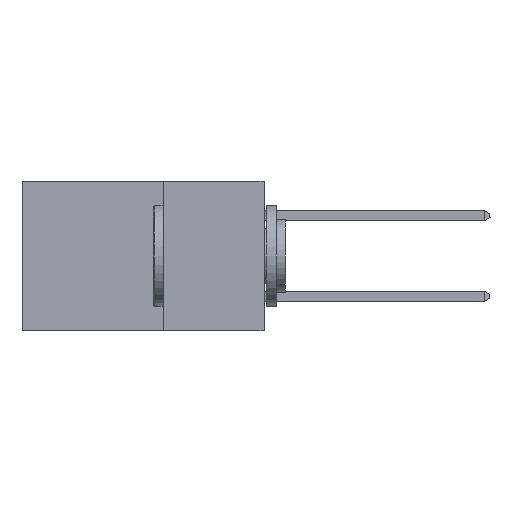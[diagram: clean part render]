
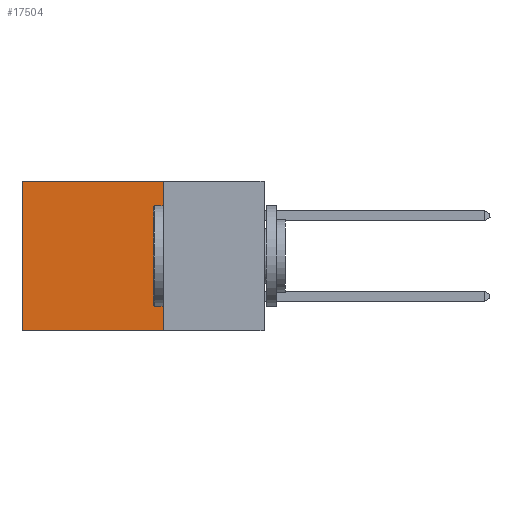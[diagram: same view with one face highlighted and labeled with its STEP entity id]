
A CAD part, left-side view. The second image highlights one B-rep face of the part: STEP entity #17504.
In plain terms, the highlighted planar face has unit normal (-1, 0, 0).
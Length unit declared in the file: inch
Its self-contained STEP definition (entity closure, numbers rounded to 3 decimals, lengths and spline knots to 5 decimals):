
#246 = CARTESIAN_POINT ( 'NONE',  ( 0.298, 0.6, 0. ) ) ;
#4098 = DIRECTION ( 'NONE',  ( 0., 1., 0. ) ) ;
#4342 = LINE ( 'NONE', #7445, #29197 ) ;
#4392 = CARTESIAN_POINT ( 'NONE',  ( 0.298, 0.25, -0.37 ) ) ;
#4753 = ORIENTED_EDGE ( 'NONE', *, *, #19702, .T. ) ;
#7445 = CARTESIAN_POINT ( 'NONE',  ( 0.298, 0.25, 0. ) ) ;
#9048 = VECTOR ( 'NONE', #27090, 39.37008 ) ;
#9497 = LINE ( 'NONE', #11102, #12648 ) ;
#10678 = ORIENTED_EDGE ( 'NONE', *, *, #26498, .T. ) ;
#10908 = PLANE ( 'NONE',  #15287 ) ;
#11012 = CARTESIAN_POINT ( 'NONE',  ( 0.298, 0.25, 0. ) ) ;
#11102 = CARTESIAN_POINT ( 'NONE',  ( 0.298, 0.25, 0. ) ) ;
#12343 = EDGE_CURVE ( 'NONE', #18523, #13558, #13963, .T. ) ;
#12648 = VECTOR ( 'NONE', #4098, 39.37008 ) ;
#13558 = VERTEX_POINT ( 'NONE', #21492 ) ;
#13963 = LINE ( 'NONE', #4392, #9048 ) ;
#14681 = CARTESIAN_POINT ( 'NONE',  ( 0.298, 0.6, 0. ) ) ;
#15287 = AXIS2_PLACEMENT_3D ( 'NONE', #11012, #15636, #27094 ) ;
#15636 = DIRECTION ( 'NONE',  ( 1., 0., 0. ) ) ;
#16677 = VERTEX_POINT ( 'NONE', #14681 ) ;
#16897 = VECTOR ( 'NONE', #22634, 39.37008 ) ;
#16905 = ORIENTED_EDGE ( 'NONE', *, *, #27891, .F. ) ;
#17504 = ADVANCED_FACE ( 'NONE', ( #17761 ), #10908, .F. ) ;
#17761 = FACE_OUTER_BOUND ( 'NONE', #19404, .T. ) ;
#17885 = CARTESIAN_POINT ( 'NONE',  ( 0.298, 0.25, -0.37 ) ) ;
#18503 = ORIENTED_EDGE ( 'NONE', *, *, #12343, .F. ) ;
#18523 = VERTEX_POINT ( 'NONE', #17885 ) ;
#18918 = DIRECTION ( 'NONE',  ( 0., 0., -1. ) ) ;
#19404 = EDGE_LOOP ( 'NONE', ( #4753, #18503, #16905, #10678 ) ) ;
#19702 = EDGE_CURVE ( 'NONE', #16677, #13558, #24008, .T. ) ;
#21492 = CARTESIAN_POINT ( 'NONE',  ( 0.298, 0.6, -0.37 ) ) ;
#22634 = DIRECTION ( 'NONE',  ( 0., 0., -1. ) ) ;
#24008 = LINE ( 'NONE', #246, #16897 ) ;
#25825 = CARTESIAN_POINT ( 'NONE',  ( 0.298, 0.25, 0. ) ) ;
#26498 = EDGE_CURVE ( 'NONE', #27314, #16677, #9497, .T. ) ;
#27090 = DIRECTION ( 'NONE',  ( 0., 1., 0. ) ) ;
#27094 = DIRECTION ( 'NONE',  ( 0., 0., -1. ) ) ;
#27314 = VERTEX_POINT ( 'NONE', #25825 ) ;
#27891 = EDGE_CURVE ( 'NONE', #27314, #18523, #4342, .T. ) ;
#29197 = VECTOR ( 'NONE', #18918, 39.37008 ) ;
